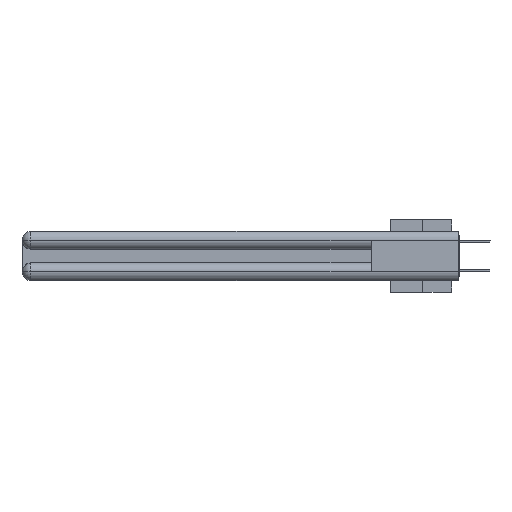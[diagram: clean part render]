
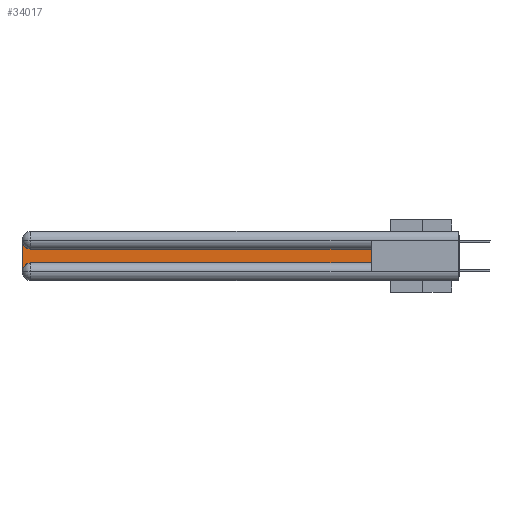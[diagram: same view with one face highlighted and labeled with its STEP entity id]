
A CAD part, left-side view. The second image highlights one B-rep face of the part: STEP entity #34017.
In plain terms, the highlighted planar face has unit normal (-1, 0, 0).
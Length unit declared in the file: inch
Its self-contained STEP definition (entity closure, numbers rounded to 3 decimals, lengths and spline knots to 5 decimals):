
#175 = VERTEX_POINT ( 'NONE', #17775 ) ;
#390 = CARTESIAN_POINT ( 'NONE',  ( 0.075, 2.94, -0.1225 ) ) ;
#605 = CARTESIAN_POINT ( 'NONE',  ( 0.075, 2.94, -0.2775 ) ) ;
#833 = EDGE_CURVE ( 'NONE', #175, #6637, #10712, .T. ) ;
#1262 = FACE_OUTER_BOUND ( 'NONE', #17094, .T. ) ;
#3209 = VERTEX_POINT ( 'NONE', #32448 ) ;
#3327 = EDGE_CURVE ( 'NONE', #6637, #16275, #9985, .T. ) ;
#4056 = VERTEX_POINT ( 'NONE', #32301 ) ;
#4620 = DIRECTION ( 'NONE',  ( 0., 0., -1. ) ) ;
#5175 = EDGE_CURVE ( 'NONE', #3209, #175, #24594, .T. ) ;
#6637 = VERTEX_POINT ( 'NONE', #34068 ) ;
#6674 = DIRECTION ( 'NONE',  ( 0., 0., -1. ) ) ;
#6840 = DIRECTION ( 'NONE',  ( 0., 1., 0. ) ) ;
#7786 = VECTOR ( 'NONE', #6840, 39.37008 ) ;
#8490 = AXIS2_PLACEMENT_3D ( 'NONE', #605, #32715, #26386 ) ;
#9663 = CARTESIAN_POINT ( 'NONE',  ( 0.075, 3., -0.0625 ) ) ;
#9985 = LINE ( 'NONE', #20041, #7786 ) ;
#10712 = LINE ( 'NONE', #16376, #30280 ) ;
#13499 = DIRECTION ( 'NONE',  ( 0., 0., -1. ) ) ;
#16275 = VERTEX_POINT ( 'NONE', #390 ) ;
#16376 = CARTESIAN_POINT ( 'NONE',  ( 0.075, 0.6, -0.2175 ) ) ;
#17001 = ORIENTED_EDGE ( 'NONE', *, *, #5175, .T. ) ;
#17094 = EDGE_LOOP ( 'NONE', ( #22828, #25429, #25498, #40030, #17001, #31135 ) ) ;
#17508 = VECTOR ( 'NONE', #34269, 39.37008 ) ;
#17666 = EDGE_CURVE ( 'NONE', #4056, #3209, #26588, .T. ) ;
#17775 = CARTESIAN_POINT ( 'NONE',  ( 0.075, 0.6, -0.2175 ) ) ;
#19522 = DIRECTION ( 'NONE',  ( 0., 0., 1. ) ) ;
#20018 = EDGE_CURVE ( 'NONE', #35490, #4056, #26921, .T. ) ;
#20041 = CARTESIAN_POINT ( 'NONE',  ( 0.075, 0.6, -0.1225 ) ) ;
#20825 = AXIS2_PLACEMENT_3D ( 'NONE', #22205, #38835, #6674 ) ;
#20955 = PLANE ( 'NONE',  #21235 ) ;
#21235 = AXIS2_PLACEMENT_3D ( 'NONE', #39924, #39717, #4620 ) ;
#22205 = CARTESIAN_POINT ( 'NONE',  ( 0.075, 2.94, -0.0625 ) ) ;
#22828 = ORIENTED_EDGE ( 'NONE', *, *, #3327, .T. ) ;
#24184 = CARTESIAN_POINT ( 'NONE',  ( 0.075, 0.6, -0.2175 ) ) ;
#24594 = LINE ( 'NONE', #24184, #17508 ) ;
#24804 = VECTOR ( 'NONE', #13499, 39.37008 ) ;
#25429 = ORIENTED_EDGE ( 'NONE', *, *, #25962, .T. ) ;
#25498 = ORIENTED_EDGE ( 'NONE', *, *, #20018, .T. ) ;
#25962 = EDGE_CURVE ( 'NONE', #16275, #35490, #33574, .T. ) ;
#26386 = DIRECTION ( 'NONE',  ( 0., 0., -1. ) ) ;
#26588 = CIRCLE ( 'NONE', #8490, 0.06 ) ;
#26921 = LINE ( 'NONE', #39792, #24804 ) ;
#30280 = VECTOR ( 'NONE', #19522, 39.37008 ) ;
#31135 = ORIENTED_EDGE ( 'NONE', *, *, #833, .T. ) ;
#32301 = CARTESIAN_POINT ( 'NONE',  ( 0.075, 3., -0.2775 ) ) ;
#32448 = CARTESIAN_POINT ( 'NONE',  ( 0.075, 2.94, -0.2175 ) ) ;
#32715 = DIRECTION ( 'NONE',  ( 1., 0., 0. ) ) ;
#33574 = CIRCLE ( 'NONE', #20825, 0.06 ) ;
#34017 = ADVANCED_FACE ( 'NONE', ( #1262 ), #20955, .F. ) ;
#34068 = CARTESIAN_POINT ( 'NONE',  ( 0.075, 0.6, -0.1225 ) ) ;
#34269 = DIRECTION ( 'NONE',  ( 0., -1., 0. ) ) ;
#35490 = VERTEX_POINT ( 'NONE', #9663 ) ;
#38835 = DIRECTION ( 'NONE',  ( 1., 0., 0. ) ) ;
#39717 = DIRECTION ( 'NONE',  ( 1., 0., 0. ) ) ;
#39792 = CARTESIAN_POINT ( 'NONE',  ( 0.075, 3., -0.2175 ) ) ;
#39924 = CARTESIAN_POINT ( 'NONE',  ( 0.075, 3., -0.1225 ) ) ;
#40030 = ORIENTED_EDGE ( 'NONE', *, *, #17666, .T. ) ;
